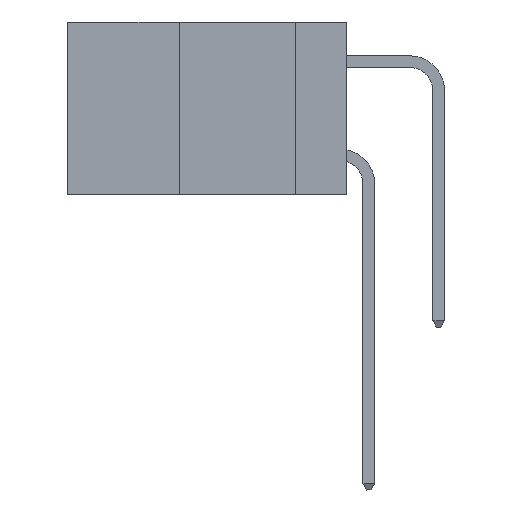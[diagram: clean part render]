
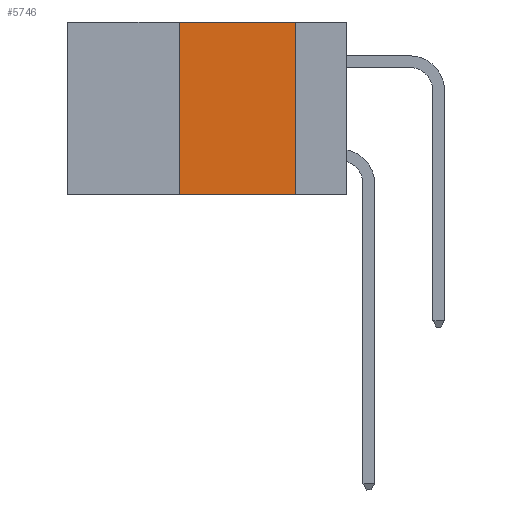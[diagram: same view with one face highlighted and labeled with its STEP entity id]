
A CAD part, left-side view. The second image highlights one B-rep face of the part: STEP entity #5746.
In plain terms, the highlighted planar face has unit normal (-1, 0, 0).
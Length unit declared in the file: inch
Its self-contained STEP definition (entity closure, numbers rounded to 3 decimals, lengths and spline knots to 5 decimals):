
#1604 = EDGE_CURVE ( 'NONE', #9047, #19127, #7401, .T. ) ;
#2176 = EDGE_CURVE ( 'NONE', #3526, #19127, #16429, .T. ) ;
#2464 = VECTOR ( 'NONE', #20534, 39.37008 ) ;
#2505 = VECTOR ( 'NONE', #8504, 39.37008 ) ;
#2977 = CARTESIAN_POINT ( 'NONE',  ( 0., 0.6, 0. ) ) ;
#3526 = VERTEX_POINT ( 'NONE', #8817 ) ;
#3637 = VECTOR ( 'NONE', #22925, 39.37008 ) ;
#5324 = ORIENTED_EDGE ( 'NONE', *, *, #7626, .F. ) ;
#5326 = CARTESIAN_POINT ( 'NONE',  ( 0., 0.36, -0.37 ) ) ;
#5746 = ADVANCED_FACE ( 'NONE', ( #10985 ), #15761, .F. ) ;
#6571 = CARTESIAN_POINT ( 'NONE',  ( 0., 0.11, -0.37 ) ) ;
#6708 = DIRECTION ( 'NONE',  ( 0., 0., -1. ) ) ;
#7401 = LINE ( 'NONE', #22118, #2464 ) ;
#7626 = EDGE_CURVE ( 'NONE', #9047, #14396, #22353, .T. ) ;
#8022 = LINE ( 'NONE', #12123, #2505 ) ;
#8504 = DIRECTION ( 'NONE',  ( 0., -1., 0. ) ) ;
#8817 = CARTESIAN_POINT ( 'NONE',  ( 0., 0.11, 0. ) ) ;
#9047 = VERTEX_POINT ( 'NONE', #5326 ) ;
#10162 = EDGE_CURVE ( 'NONE', #14396, #3526, #8022, .T. ) ;
#10410 = AXIS2_PLACEMENT_3D ( 'NONE', #2977, #17577, #6708 ) ;
#10985 = FACE_OUTER_BOUND ( 'NONE', #16346, .T. ) ;
#12123 = CARTESIAN_POINT ( 'NONE',  ( 0., 0.6, 0. ) ) ;
#14244 = CARTESIAN_POINT ( 'NONE',  ( 0., 0.36, 0. ) ) ;
#14363 = ORIENTED_EDGE ( 'NONE', *, *, #2176, .F. ) ;
#14396 = VERTEX_POINT ( 'NONE', #14244 ) ;
#15135 = DIRECTION ( 'NONE',  ( 0., 0., -1. ) ) ;
#15761 = PLANE ( 'NONE',  #10410 ) ;
#16346 = EDGE_LOOP ( 'NONE', ( #14363, #17722, #5324, #17070 ) ) ;
#16429 = LINE ( 'NONE', #21635, #20062 ) ;
#17070 = ORIENTED_EDGE ( 'NONE', *, *, #1604, .T. ) ;
#17577 = DIRECTION ( 'NONE',  ( 1., 0., 0. ) ) ;
#17722 = ORIENTED_EDGE ( 'NONE', *, *, #10162, .F. ) ;
#19127 = VERTEX_POINT ( 'NONE', #6571 ) ;
#19384 = CARTESIAN_POINT ( 'NONE',  ( 0., 0.36, 0. ) ) ;
#20062 = VECTOR ( 'NONE', #15135, 39.37008 ) ;
#20534 = DIRECTION ( 'NONE',  ( 0., -1., 0. ) ) ;
#21635 = CARTESIAN_POINT ( 'NONE',  ( 0., 0.11, 0. ) ) ;
#22118 = CARTESIAN_POINT ( 'NONE',  ( 0., 0.6, -0.37 ) ) ;
#22353 = LINE ( 'NONE', #19384, #3637 ) ;
#22925 = DIRECTION ( 'NONE',  ( 0., 0., 1. ) ) ;
